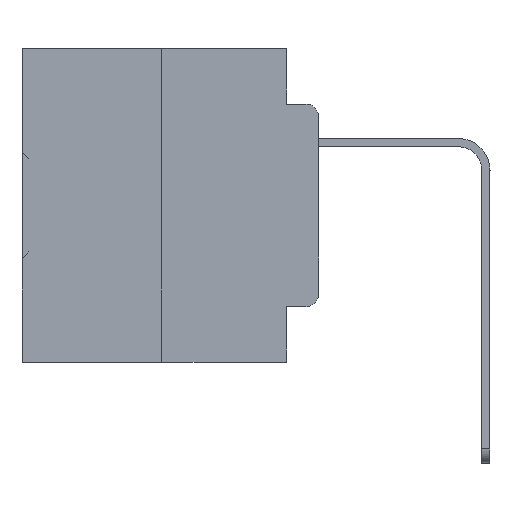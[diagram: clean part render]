
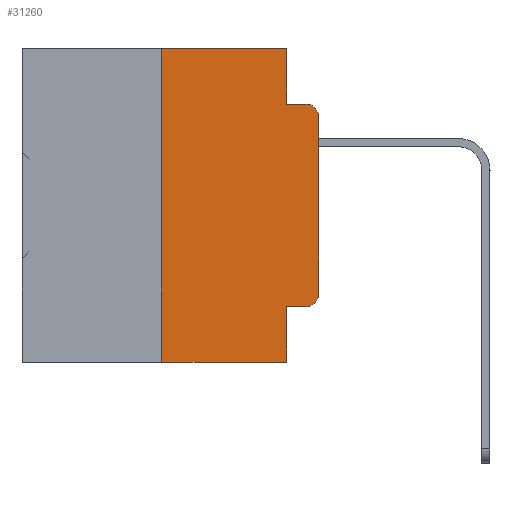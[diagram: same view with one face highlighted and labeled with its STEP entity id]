
A CAD part, left-side view. The second image highlights one B-rep face of the part: STEP entity #31260.
In plain terms, the highlighted planar face has unit normal (-1, 0, 0).
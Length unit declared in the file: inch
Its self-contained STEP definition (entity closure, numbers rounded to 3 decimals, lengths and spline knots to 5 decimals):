
#68 = CARTESIAN_POINT ( 'NONE',  ( 0., 0.473, 0. ) ) ;
#314 = ORIENTED_EDGE ( 'NONE', *, *, #31930, .T. ) ;
#612 = VERTEX_POINT ( 'NONE', #14799 ) ;
#823 = DIRECTION ( 'NONE',  ( 0., 0., 1. ) ) ;
#1378 = LINE ( 'NONE', #35720, #31731 ) ;
#1757 = CARTESIAN_POINT ( 'NONE',  ( 0., 0.02, -0.3915 ) ) ;
#1772 = EDGE_CURVE ( 'NONE', #12733, #25244, #33200, .T. ) ;
#1784 = CARTESIAN_POINT ( 'NONE',  ( 0., 0., -0.3915 ) ) ;
#1868 = ORIENTED_EDGE ( 'NONE', *, *, #1772, .F. ) ;
#2649 = CARTESIAN_POINT ( 'NONE',  ( 0., 0.02, -0.1085 ) ) ;
#5576 = ORIENTED_EDGE ( 'NONE', *, *, #29069, .T. ) ;
#6355 = VERTEX_POINT ( 'NONE', #19399 ) ;
#6421 = CARTESIAN_POINT ( 'NONE',  ( 0., 0., -0.1085 ) ) ;
#8146 = VERTEX_POINT ( 'NONE', #14736 ) ;
#8323 = DIRECTION ( 'NONE',  ( -1., 0., 0. ) ) ;
#8453 = ORIENTED_EDGE ( 'NONE', *, *, #16257, .F. ) ;
#8711 = DIRECTION ( 'NONE',  ( 0., -1., 0. ) ) ;
#8754 = CARTESIAN_POINT ( 'NONE',  ( 0., 0.25, 0. ) ) ;
#8793 = ORIENTED_EDGE ( 'NONE', *, *, #9239, .F. ) ;
#9239 = EDGE_CURVE ( 'NONE', #18933, #30681, #16147, .T. ) ;
#9542 = DIRECTION ( 'NONE',  ( 0., 0., -1. ) ) ;
#9655 = AXIS2_PLACEMENT_3D ( 'NONE', #19324, #22258, #31101 ) ;
#9674 = CARTESIAN_POINT ( 'NONE',  ( 0., 0.25, -0.5 ) ) ;
#10535 = DIRECTION ( 'NONE',  ( 0., 0., -1. ) ) ;
#11336 = VECTOR ( 'NONE', #8711, 39.37008 ) ;
#12733 = VERTEX_POINT ( 'NONE', #9674 ) ;
#13473 = VERTEX_POINT ( 'NONE', #6421 ) ;
#13593 = CARTESIAN_POINT ( 'NONE',  ( 0., 0.473, -0.5 ) ) ;
#14726 = LINE ( 'NONE', #37285, #20734 ) ;
#14736 = CARTESIAN_POINT ( 'NONE',  ( 0., 0.051, 0. ) ) ;
#14799 = CARTESIAN_POINT ( 'NONE',  ( 0., 0.02, -0.4115 ) ) ;
#16147 = LINE ( 'NONE', #28859, #18455 ) ;
#16257 = EDGE_CURVE ( 'NONE', #25244, #8146, #16376, .T. ) ;
#16284 = VECTOR ( 'NONE', #28619, 39.37008 ) ;
#16376 = LINE ( 'NONE', #68, #11336 ) ;
#16584 = CARTESIAN_POINT ( 'NONE',  ( 0., 0.25, 0. ) ) ;
#16646 = CARTESIAN_POINT ( 'NONE',  ( 0., 0.051, -0.5 ) ) ;
#16673 = LINE ( 'NONE', #33090, #29961 ) ;
#16803 = ORIENTED_EDGE ( 'NONE', *, *, #22557, .F. ) ;
#17702 = VERTEX_POINT ( 'NONE', #1784 ) ;
#18455 = VECTOR ( 'NONE', #29232, 39.37008 ) ;
#18933 = VERTEX_POINT ( 'NONE', #36988 ) ;
#19324 = CARTESIAN_POINT ( 'NONE',  ( 0., 0.473, 0. ) ) ;
#19399 = CARTESIAN_POINT ( 'NONE',  ( 0., 0.051, -0.0885 ) ) ;
#19657 = DIRECTION ( 'NONE',  ( 0., -1., 0. ) ) ;
#19734 = CIRCLE ( 'NONE', #23898, 0.02 ) ;
#20213 = ORIENTED_EDGE ( 'NONE', *, *, #29333, .F. ) ;
#20245 = CARTESIAN_POINT ( 'NONE',  ( 0., 0.02, -0.0885 ) ) ;
#20469 = CIRCLE ( 'NONE', #30353, 0.02 ) ;
#20734 = VECTOR ( 'NONE', #22594, 39.37008 ) ;
#21315 = ORIENTED_EDGE ( 'NONE', *, *, #34252, .T. ) ;
#22258 = DIRECTION ( 'NONE',  ( 1., 0., 0. ) ) ;
#22557 = EDGE_CURVE ( 'NONE', #8146, #6355, #16673, .T. ) ;
#22594 = DIRECTION ( 'NONE',  ( 0., -1., 0. ) ) ;
#23898 = AXIS2_PLACEMENT_3D ( 'NONE', #1757, #28476, #10535 ) ;
#24595 = VERTEX_POINT ( 'NONE', #20245 ) ;
#24927 = PLANE ( 'NONE',  #9655 ) ;
#25244 = VERTEX_POINT ( 'NONE', #8754 ) ;
#26265 = ORIENTED_EDGE ( 'NONE', *, *, #34138, .T. ) ;
#26890 = LINE ( 'NONE', #13593, #34620 ) ;
#28476 = DIRECTION ( 'NONE',  ( -1., 0., 0. ) ) ;
#28619 = DIRECTION ( 'NONE',  ( 0., 0., 1. ) ) ;
#28859 = CARTESIAN_POINT ( 'NONE',  ( 0., 0.051, 0. ) ) ;
#29069 = EDGE_CURVE ( 'NONE', #17702, #13473, #1378, .T. ) ;
#29232 = DIRECTION ( 'NONE',  ( 0., 0., -1. ) ) ;
#29333 = EDGE_CURVE ( 'NONE', #6355, #24595, #29415, .T. ) ;
#29415 = LINE ( 'NONE', #30690, #33051 ) ;
#29961 = VECTOR ( 'NONE', #9542, 39.37008 ) ;
#30353 = AXIS2_PLACEMENT_3D ( 'NONE', #2649, #8323, #35107 ) ;
#30490 = ORIENTED_EDGE ( 'NONE', *, *, #37277, .T. ) ;
#30681 = VERTEX_POINT ( 'NONE', #16646 ) ;
#30690 = CARTESIAN_POINT ( 'NONE',  ( 0., 0.051, -0.0885 ) ) ;
#30839 = EDGE_LOOP ( 'NONE', ( #5576, #21315, #20213, #16803, #8453, #1868, #26265, #8793, #30490, #314 ) ) ;
#31101 = DIRECTION ( 'NONE',  ( 0., 0., -1. ) ) ;
#31260 = ADVANCED_FACE ( 'NONE', ( #37940 ), #24927, .F. ) ;
#31731 = VECTOR ( 'NONE', #823, 39.37008 ) ;
#31930 = EDGE_CURVE ( 'NONE', #612, #17702, #19734, .T. ) ;
#33051 = VECTOR ( 'NONE', #36447, 39.37008 ) ;
#33090 = CARTESIAN_POINT ( 'NONE',  ( 0., 0.051, 0. ) ) ;
#33200 = LINE ( 'NONE', #16584, #16284 ) ;
#34138 = EDGE_CURVE ( 'NONE', #12733, #30681, #26890, .T. ) ;
#34252 = EDGE_CURVE ( 'NONE', #13473, #24595, #20469, .T. ) ;
#34620 = VECTOR ( 'NONE', #19657, 39.37008 ) ;
#35107 = DIRECTION ( 'NONE',  ( 0., 0., -1. ) ) ;
#35720 = CARTESIAN_POINT ( 'NONE',  ( 0., 0., 0. ) ) ;
#36447 = DIRECTION ( 'NONE',  ( 0., -1., 0. ) ) ;
#36988 = CARTESIAN_POINT ( 'NONE',  ( 0., 0.051, -0.4115 ) ) ;
#37277 = EDGE_CURVE ( 'NONE', #18933, #612, #14726, .T. ) ;
#37285 = CARTESIAN_POINT ( 'NONE',  ( 0., 0.051, -0.4115 ) ) ;
#37940 = FACE_OUTER_BOUND ( 'NONE', #30839, .T. ) ;
